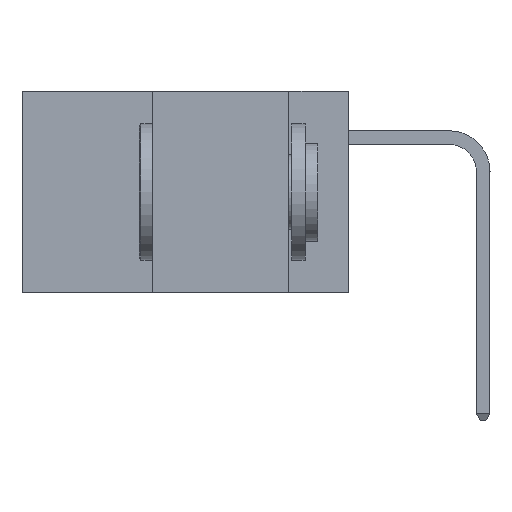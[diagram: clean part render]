
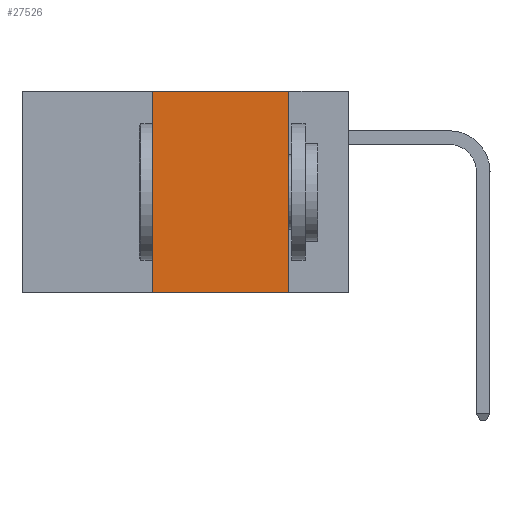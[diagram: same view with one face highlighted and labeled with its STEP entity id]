
A CAD part, left-side view. The second image highlights one B-rep face of the part: STEP entity #27526.
In plain terms, the highlighted planar face has unit normal (-1, 0, 0).
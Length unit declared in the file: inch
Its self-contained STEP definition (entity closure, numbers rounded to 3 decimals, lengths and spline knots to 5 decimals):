
#1363 = VERTEX_POINT ( 'NONE', #20123 ) ;
#2797 = PLANE ( 'NONE',  #16727 ) ;
#3104 = ORIENTED_EDGE ( 'NONE', *, *, #33725, .F. ) ;
#4287 = VECTOR ( 'NONE', #16292, 39.37008 ) ;
#4914 = LINE ( 'NONE', #10242, #11667 ) ;
#6648 = CARTESIAN_POINT ( 'NONE',  ( 0., 0.11, 0. ) ) ;
#7117 = ORIENTED_EDGE ( 'NONE', *, *, #8047, .F. ) ;
#7421 = VECTOR ( 'NONE', #15453, 39.37008 ) ;
#7908 = LINE ( 'NONE', #20900, #22243 ) ;
#8047 = EDGE_CURVE ( 'NONE', #14208, #13083, #7908, .T. ) ;
#8704 = CARTESIAN_POINT ( 'NONE',  ( 0., 0.36, -0.37 ) ) ;
#10242 = CARTESIAN_POINT ( 'NONE',  ( 0., 0.6, 0. ) ) ;
#11495 = CARTESIAN_POINT ( 'NONE',  ( 0., 0.6, 0. ) ) ;
#11667 = VECTOR ( 'NONE', #13131, 39.37008 ) ;
#12596 = EDGE_CURVE ( 'NONE', #1363, #14208, #4914, .T. ) ;
#12851 = LINE ( 'NONE', #36282, #4287 ) ;
#13083 = VERTEX_POINT ( 'NONE', #15109 ) ;
#13131 = DIRECTION ( 'NONE',  ( 0., -1., 0. ) ) ;
#14208 = VERTEX_POINT ( 'NONE', #6648 ) ;
#14387 = DIRECTION ( 'NONE',  ( 0., 0., -1. ) ) ;
#15109 = CARTESIAN_POINT ( 'NONE',  ( 0., 0.11, -0.37 ) ) ;
#15453 = DIRECTION ( 'NONE',  ( 0., 0., 1. ) ) ;
#16292 = DIRECTION ( 'NONE',  ( 0., -1., 0. ) ) ;
#16727 = AXIS2_PLACEMENT_3D ( 'NONE', #11495, #31552, #14387 ) ;
#18928 = VERTEX_POINT ( 'NONE', #8704 ) ;
#20123 = CARTESIAN_POINT ( 'NONE',  ( 0., 0.36, 0. ) ) ;
#20134 = ORIENTED_EDGE ( 'NONE', *, *, #29468, .T. ) ;
#20900 = CARTESIAN_POINT ( 'NONE',  ( 0., 0.11, 0. ) ) ;
#22243 = VECTOR ( 'NONE', #23776, 39.37008 ) ;
#23776 = DIRECTION ( 'NONE',  ( 0., 0., -1. ) ) ;
#25946 = FACE_OUTER_BOUND ( 'NONE', #35664, .T. ) ;
#26396 = ORIENTED_EDGE ( 'NONE', *, *, #12596, .F. ) ;
#27526 = ADVANCED_FACE ( 'NONE', ( #25946 ), #2797, .F. ) ;
#29468 = EDGE_CURVE ( 'NONE', #18928, #13083, #12851, .T. ) ;
#29744 = CARTESIAN_POINT ( 'NONE',  ( 0., 0.36, 0. ) ) ;
#31552 = DIRECTION ( 'NONE',  ( 1., 0., 0. ) ) ;
#33725 = EDGE_CURVE ( 'NONE', #18928, #1363, #36079, .T. ) ;
#35664 = EDGE_LOOP ( 'NONE', ( #7117, #26396, #3104, #20134 ) ) ;
#36079 = LINE ( 'NONE', #29744, #7421 ) ;
#36282 = CARTESIAN_POINT ( 'NONE',  ( 0., 0.6, -0.37 ) ) ;
